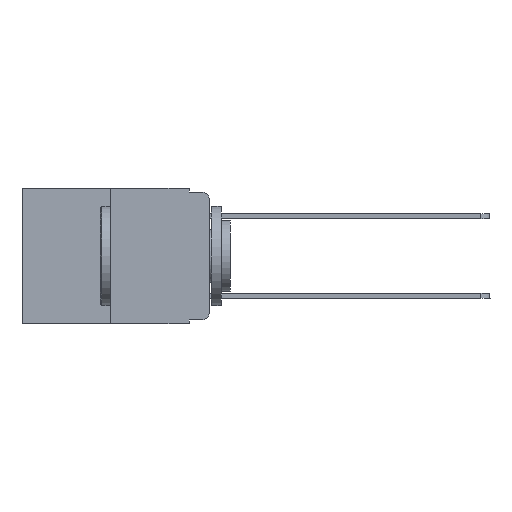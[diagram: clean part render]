
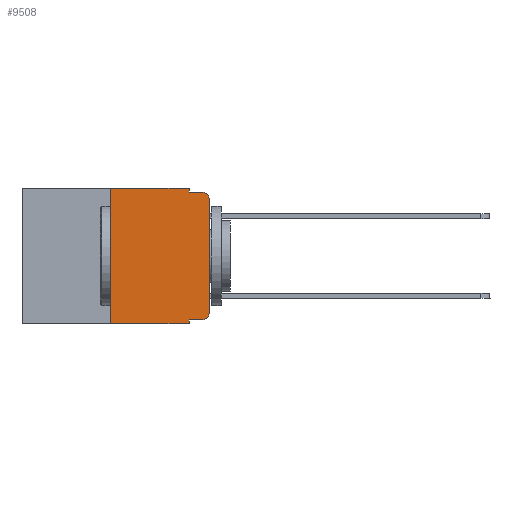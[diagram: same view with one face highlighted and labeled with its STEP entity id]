
A CAD part, left-side view. The second image highlights one B-rep face of the part: STEP entity #9508.
In plain terms, the highlighted planar face has unit normal (-1, 0, 0).
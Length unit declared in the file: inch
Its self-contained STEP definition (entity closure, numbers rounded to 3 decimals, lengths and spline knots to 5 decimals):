
#529 = CARTESIAN_POINT ( 'NONE',  ( 0., 0.051, 0. ) ) ;
#705 = DIRECTION ( 'NONE',  ( -1., 0., 0. ) ) ;
#882 = VECTOR ( 'NONE', #11562, 39.37008 ) ;
#975 = DIRECTION ( 'NONE',  ( 0., 0., 1. ) ) ;
#1112 = LINE ( 'NONE', #4511, #10113 ) ;
#1153 = VERTEX_POINT ( 'NONE', #6594 ) ;
#1519 = ORIENTED_EDGE ( 'NONE', *, *, #4974, .F. ) ;
#1942 = CARTESIAN_POINT ( 'NONE',  ( 0., 0.02, -0.01 ) ) ;
#2246 = CARTESIAN_POINT ( 'NONE',  ( 0., 0.25, -0.343 ) ) ;
#2306 = VECTOR ( 'NONE', #21136, 39.37008 ) ;
#2919 = LINE ( 'NONE', #21340, #18845 ) ;
#3134 = AXIS2_PLACEMENT_3D ( 'NONE', #7480, #705, #14359 ) ;
#4032 = LINE ( 'NONE', #5785, #5600 ) ;
#4060 = VECTOR ( 'NONE', #15761, 39.37008 ) ;
#4511 = CARTESIAN_POINT ( 'NONE',  ( 0., 0.473, 0. ) ) ;
#4974 = EDGE_CURVE ( 'NONE', #5854, #7149, #10377, .T. ) ;
#5238 = CIRCLE ( 'NONE', #3134, 0.02 ) ;
#5483 = AXIS2_PLACEMENT_3D ( 'NONE', #18173, #19596, #19921 ) ;
#5600 = VECTOR ( 'NONE', #975, 39.37008 ) ;
#5785 = CARTESIAN_POINT ( 'NONE',  ( 0., 0.25, 0. ) ) ;
#5854 = VERTEX_POINT ( 'NONE', #5920 ) ;
#5920 = CARTESIAN_POINT ( 'NONE',  ( 0., 0.051, 0. ) ) ;
#6093 = LINE ( 'NONE', #11139, #2306 ) ;
#6594 = CARTESIAN_POINT ( 'NONE',  ( 0., 0., -0.313 ) ) ;
#7082 = LINE ( 'NONE', #12101, #19446 ) ;
#7149 = VERTEX_POINT ( 'NONE', #8687 ) ;
#7283 = ORIENTED_EDGE ( 'NONE', *, *, #13186, .F. ) ;
#7326 = ORIENTED_EDGE ( 'NONE', *, *, #16654, .F. ) ;
#7480 = CARTESIAN_POINT ( 'NONE',  ( 0., 0.02, -0.03 ) ) ;
#7762 = FACE_OUTER_BOUND ( 'NONE', #10970, .T. ) ;
#7790 = VERTEX_POINT ( 'NONE', #14727 ) ;
#7964 = CARTESIAN_POINT ( 'NONE',  ( 0., 0.051, -0.333 ) ) ;
#8687 = CARTESIAN_POINT ( 'NONE',  ( 0., 0.051, -0.01 ) ) ;
#8707 = LINE ( 'NONE', #10342, #4060 ) ;
#9355 = CARTESIAN_POINT ( 'NONE',  ( 0., 0., -0.03 ) ) ;
#9508 = ADVANCED_FACE ( 'NONE', ( #7762 ), #17793, .F. ) ;
#9851 = ORIENTED_EDGE ( 'NONE', *, *, #18825, .T. ) ;
#10113 = VECTOR ( 'NONE', #11179, 39.37008 ) ;
#10210 = EDGE_CURVE ( 'NONE', #10341, #14448, #14809, .T. ) ;
#10341 = VERTEX_POINT ( 'NONE', #2246 ) ;
#10342 = CARTESIAN_POINT ( 'NONE',  ( 0., 0.051, -0.01 ) ) ;
#10377 = LINE ( 'NONE', #529, #20126 ) ;
#10576 = VERTEX_POINT ( 'NONE', #19911 ) ;
#10970 = EDGE_LOOP ( 'NONE', ( #15803, #13451, #7283, #1519, #7326, #11617, #19079, #20437, #9851, #17479 ) ) ;
#11139 = CARTESIAN_POINT ( 'NONE',  ( 0., 0., 0. ) ) ;
#11179 = DIRECTION ( 'NONE',  ( 0., -1., 0. ) ) ;
#11293 = EDGE_CURVE ( 'NONE', #1153, #18794, #6093, .T. ) ;
#11562 = DIRECTION ( 'NONE',  ( 0., -1., 0. ) ) ;
#11617 = ORIENTED_EDGE ( 'NONE', *, *, #18223, .F. ) ;
#12101 = CARTESIAN_POINT ( 'NONE',  ( 0., 0.051, 0. ) ) ;
#12643 = DIRECTION ( 'NONE',  ( 0., -1., 0. ) ) ;
#13186 = EDGE_CURVE ( 'NONE', #7149, #18548, #8707, .T. ) ;
#13451 = ORIENTED_EDGE ( 'NONE', *, *, #16267, .T. ) ;
#14107 = AXIS2_PLACEMENT_3D ( 'NONE', #14421, #21475, #14736 ) ;
#14359 = DIRECTION ( 'NONE',  ( 0., 0., -1. ) ) ;
#14421 = CARTESIAN_POINT ( 'NONE',  ( 0., 0.473, 0. ) ) ;
#14448 = VERTEX_POINT ( 'NONE', #17750 ) ;
#14727 = CARTESIAN_POINT ( 'NONE',  ( 0., 0.25, 0. ) ) ;
#14736 = DIRECTION ( 'NONE',  ( 0., 0., -1. ) ) ;
#14809 = LINE ( 'NONE', #21446, #882 ) ;
#15706 = DIRECTION ( 'NONE',  ( 0., 0., -1. ) ) ;
#15761 = DIRECTION ( 'NONE',  ( 0., -1., 0. ) ) ;
#15803 = ORIENTED_EDGE ( 'NONE', *, *, #11293, .T. ) ;
#16267 = EDGE_CURVE ( 'NONE', #18794, #18548, #5238, .T. ) ;
#16654 = EDGE_CURVE ( 'NONE', #7790, #5854, #1112, .T. ) ;
#16998 = DIRECTION ( 'NONE',  ( 0., 0., -1. ) ) ;
#17479 = ORIENTED_EDGE ( 'NONE', *, *, #21333, .T. ) ;
#17750 = CARTESIAN_POINT ( 'NONE',  ( 0., 0.051, -0.343 ) ) ;
#17793 = PLANE ( 'NONE',  #14107 ) ;
#18173 = CARTESIAN_POINT ( 'NONE',  ( 0., 0.02, -0.313 ) ) ;
#18223 = EDGE_CURVE ( 'NONE', #10341, #7790, #4032, .T. ) ;
#18322 = VERTEX_POINT ( 'NONE', #7964 ) ;
#18548 = VERTEX_POINT ( 'NONE', #1942 ) ;
#18794 = VERTEX_POINT ( 'NONE', #9355 ) ;
#18825 = EDGE_CURVE ( 'NONE', #18322, #10576, #2919, .T. ) ;
#18845 = VECTOR ( 'NONE', #12643, 39.37008 ) ;
#19079 = ORIENTED_EDGE ( 'NONE', *, *, #10210, .T. ) ;
#19446 = VECTOR ( 'NONE', #16998, 39.37008 ) ;
#19596 = DIRECTION ( 'NONE',  ( -1., 0., 0. ) ) ;
#19911 = CARTESIAN_POINT ( 'NONE',  ( 0., 0.02, -0.333 ) ) ;
#19921 = DIRECTION ( 'NONE',  ( 0., 0., -1. ) ) ;
#20126 = VECTOR ( 'NONE', #15706, 39.37008 ) ;
#20437 = ORIENTED_EDGE ( 'NONE', *, *, #21086, .F. ) ;
#20451 = CIRCLE ( 'NONE', #5483, 0.02 ) ;
#21086 = EDGE_CURVE ( 'NONE', #18322, #14448, #7082, .T. ) ;
#21136 = DIRECTION ( 'NONE',  ( 0., 0., 1. ) ) ;
#21333 = EDGE_CURVE ( 'NONE', #10576, #1153, #20451, .T. ) ;
#21340 = CARTESIAN_POINT ( 'NONE',  ( 0., 0.051, -0.333 ) ) ;
#21446 = CARTESIAN_POINT ( 'NONE',  ( 0., 0.473, -0.343 ) ) ;
#21475 = DIRECTION ( 'NONE',  ( 1., 0., 0. ) ) ;
